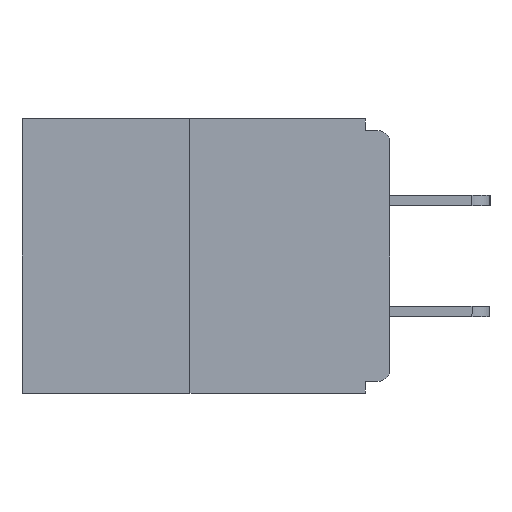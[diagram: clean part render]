
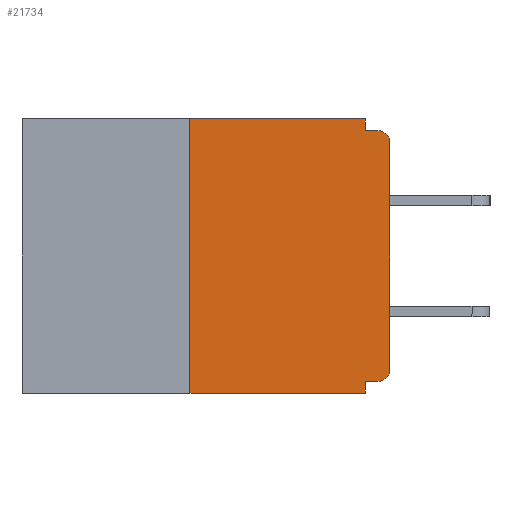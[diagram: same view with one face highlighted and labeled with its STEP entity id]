
A CAD part, left-side view. The second image highlights one B-rep face of the part: STEP entity #21734.
In plain terms, the highlighted planar face has unit normal (-1, 0, 0).
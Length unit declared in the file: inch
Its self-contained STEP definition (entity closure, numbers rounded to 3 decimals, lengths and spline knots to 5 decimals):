
#237 = EDGE_CURVE ( 'NONE', #14467, #5937, #25285, .T. ) ;
#824 = LINE ( 'NONE', #19293, #19291 ) ;
#1142 = CARTESIAN_POINT ( 'NONE',  ( 0., 0.031, 0. ) ) ;
#1185 = AXIS2_PLACEMENT_3D ( 'NONE', #10390, #17109, #14917 ) ;
#1374 = VERTEX_POINT ( 'NONE', #20596 ) ;
#1946 = DIRECTION ( 'NONE',  ( 0., 0., 1. ) ) ;
#2296 = VERTEX_POINT ( 'NONE', #13994 ) ;
#2475 = EDGE_CURVE ( 'NONE', #2296, #6537, #16624, .T. ) ;
#2834 = CARTESIAN_POINT ( 'NONE',  ( 0., 0., -0.03 ) ) ;
#2846 = CIRCLE ( 'NONE', #12746, 0.015 ) ;
#3547 = FACE_OUTER_BOUND ( 'NONE', #11977, .T. ) ;
#3580 = VECTOR ( 'NONE', #14974, 39.37008 ) ;
#3604 = DIRECTION ( 'NONE',  ( 0., -1., 0. ) ) ;
#3956 = CARTESIAN_POINT ( 'NONE',  ( 0., 0., -0.328 ) ) ;
#4335 = CARTESIAN_POINT ( 'NONE',  ( 0., 0.25, 0. ) ) ;
#4753 = VECTOR ( 'NONE', #5980, 39.37008 ) ;
#4761 = CARTESIAN_POINT ( 'NONE',  ( 0., 0.25, 0. ) ) ;
#4957 = ORIENTED_EDGE ( 'NONE', *, *, #2475, .F. ) ;
#5054 = ORIENTED_EDGE ( 'NONE', *, *, #237, .T. ) ;
#5689 = VECTOR ( 'NONE', #27320, 39.37008 ) ;
#5937 = VERTEX_POINT ( 'NONE', #2834 ) ;
#5980 = DIRECTION ( 'NONE',  ( 0., 1., 0. ) ) ;
#6537 = VERTEX_POINT ( 'NONE', #8684 ) ;
#6668 = CARTESIAN_POINT ( 'NONE',  ( 0., 0.031, 0. ) ) ;
#7038 = DIRECTION ( 'NONE',  ( 0., 0., -1. ) ) ;
#7133 = LINE ( 'NONE', #4335, #15358 ) ;
#7341 = ORIENTED_EDGE ( 'NONE', *, *, #26747, .F. ) ;
#8253 = ORIENTED_EDGE ( 'NONE', *, *, #8977, .T. ) ;
#8407 = DIRECTION ( 'NONE',  ( 0., 0., 1. ) ) ;
#8684 = CARTESIAN_POINT ( 'NONE',  ( 0., 0.031, -0.328 ) ) ;
#8977 = EDGE_CURVE ( 'NONE', #22545, #16964, #21758, .T. ) ;
#9325 = EDGE_CURVE ( 'NONE', #22545, #11911, #7133, .T. ) ;
#10236 = CARTESIAN_POINT ( 'NONE',  ( 0., 0.031, -0.015 ) ) ;
#10390 = CARTESIAN_POINT ( 'NONE',  ( 0., 0.46, 0. ) ) ;
#11347 = CARTESIAN_POINT ( 'NONE',  ( 0., 0., -0.313 ) ) ;
#11621 = CARTESIAN_POINT ( 'NONE',  ( 0., 0.031, -0.343 ) ) ;
#11911 = VERTEX_POINT ( 'NONE', #4761 ) ;
#11977 = EDGE_LOOP ( 'NONE', ( #15032, #18892, #8253, #24329, #4957, #25793, #5054, #14979, #21232, #7341 ) ) ;
#11983 = VERTEX_POINT ( 'NONE', #1142 ) ;
#12293 = EDGE_CURVE ( 'NONE', #11911, #11983, #21613, .T. ) ;
#12576 = EDGE_CURVE ( 'NONE', #6537, #16964, #824, .T. ) ;
#12746 = AXIS2_PLACEMENT_3D ( 'NONE', #14296, #14402, #18626 ) ;
#13994 = CARTESIAN_POINT ( 'NONE',  ( 0., 0.015, -0.328 ) ) ;
#14156 = EDGE_CURVE ( 'NONE', #22121, #1374, #25448, .T. ) ;
#14296 = CARTESIAN_POINT ( 'NONE',  ( 0., 0.015, -0.03 ) ) ;
#14402 = DIRECTION ( 'NONE',  ( -1., 0., 0. ) ) ;
#14467 = VERTEX_POINT ( 'NONE', #11347 ) ;
#14704 = VECTOR ( 'NONE', #15887, 39.37008 ) ;
#14878 = CARTESIAN_POINT ( 'NONE',  ( 0., 0., -0.015 ) ) ;
#14917 = DIRECTION ( 'NONE',  ( 0., 0., -1. ) ) ;
#14974 = DIRECTION ( 'NONE',  ( 0., 0., -1. ) ) ;
#14979 = ORIENTED_EDGE ( 'NONE', *, *, #15990, .T. ) ;
#15032 = ORIENTED_EDGE ( 'NONE', *, *, #12293, .F. ) ;
#15358 = VECTOR ( 'NONE', #1946, 39.37008 ) ;
#15887 = DIRECTION ( 'NONE',  ( 0., -1., 0. ) ) ;
#15990 = EDGE_CURVE ( 'NONE', #5937, #1374, #2846, .T. ) ;
#16624 = LINE ( 'NONE', #3956, #4753 ) ;
#16964 = VERTEX_POINT ( 'NONE', #11621 ) ;
#17109 = DIRECTION ( 'NONE',  ( 1., 0., 0. ) ) ;
#17497 = CARTESIAN_POINT ( 'NONE',  ( 0., 0.015, -0.313 ) ) ;
#17688 = DIRECTION ( 'NONE',  ( -1., 0., 0. ) ) ;
#18350 = VECTOR ( 'NONE', #8407, 39.37008 ) ;
#18626 = DIRECTION ( 'NONE',  ( 0., 0., -1. ) ) ;
#18892 = ORIENTED_EDGE ( 'NONE', *, *, #9325, .F. ) ;
#19004 = CARTESIAN_POINT ( 'NONE',  ( 0., 0., 0. ) ) ;
#19291 = VECTOR ( 'NONE', #7038, 39.37008 ) ;
#19293 = CARTESIAN_POINT ( 'NONE',  ( 0., 0.031, -0.343 ) ) ;
#20046 = CARTESIAN_POINT ( 'NONE',  ( 0., 0.25, -0.343 ) ) ;
#20596 = CARTESIAN_POINT ( 'NONE',  ( 0., 0.015, -0.015 ) ) ;
#20704 = LINE ( 'NONE', #6668, #3580 ) ;
#20981 = PLANE ( 'NONE',  #1185 ) ;
#21096 = VECTOR ( 'NONE', #3604, 39.37008 ) ;
#21232 = ORIENTED_EDGE ( 'NONE', *, *, #14156, .F. ) ;
#21307 = EDGE_CURVE ( 'NONE', #2296, #14467, #27014, .T. ) ;
#21613 = LINE ( 'NONE', #24369, #14704 ) ;
#21734 = ADVANCED_FACE ( 'NONE', ( #3547 ), #20981, .F. ) ;
#21758 = LINE ( 'NONE', #24602, #21096 ) ;
#22121 = VERTEX_POINT ( 'NONE', #10236 ) ;
#22545 = VERTEX_POINT ( 'NONE', #20046 ) ;
#22915 = AXIS2_PLACEMENT_3D ( 'NONE', #17497, #17688, #25898 ) ;
#24329 = ORIENTED_EDGE ( 'NONE', *, *, #12576, .F. ) ;
#24369 = CARTESIAN_POINT ( 'NONE',  ( 0., 0.46, 0. ) ) ;
#24602 = CARTESIAN_POINT ( 'NONE',  ( 0., 0.46, -0.343 ) ) ;
#25285 = LINE ( 'NONE', #19004, #18350 ) ;
#25448 = LINE ( 'NONE', #14878, #5689 ) ;
#25793 = ORIENTED_EDGE ( 'NONE', *, *, #21307, .T. ) ;
#25898 = DIRECTION ( 'NONE',  ( 0., 0., -1. ) ) ;
#26747 = EDGE_CURVE ( 'NONE', #11983, #22121, #20704, .T. ) ;
#27014 = CIRCLE ( 'NONE', #22915, 0.015 ) ;
#27320 = DIRECTION ( 'NONE',  ( 0., -1., 0. ) ) ;
